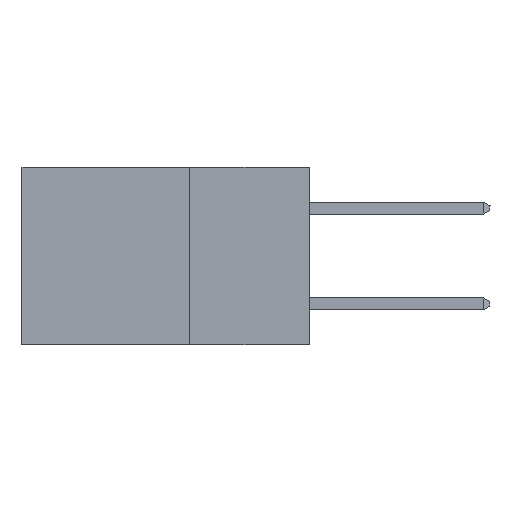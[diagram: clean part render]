
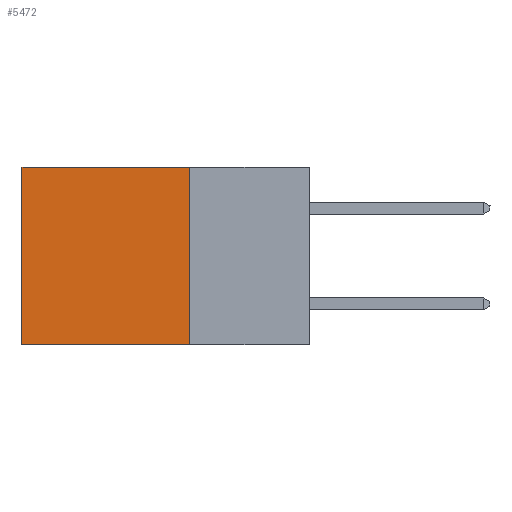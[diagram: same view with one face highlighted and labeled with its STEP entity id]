
A CAD part, left-side view. The second image highlights one B-rep face of the part: STEP entity #5472.
In plain terms, the highlighted planar face has unit normal (-1, 0, 0).
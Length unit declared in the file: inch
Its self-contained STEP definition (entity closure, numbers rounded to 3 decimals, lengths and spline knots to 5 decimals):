
#203 = LINE ( 'NONE', #6401, #4973 ) ;
#1216 = CARTESIAN_POINT ( 'NONE',  ( 0.2875, 0.25, -0.37 ) ) ;
#1405 = VERTEX_POINT ( 'NONE', #10408 ) ;
#1836 = CARTESIAN_POINT ( 'NONE',  ( 0.2875, 0.25, 0. ) ) ;
#1982 = DIRECTION ( 'NONE',  ( 1., 0., 0. ) ) ;
#2124 = VECTOR ( 'NONE', #11197, 39.37008 ) ;
#3641 = ORIENTED_EDGE ( 'NONE', *, *, #13213, .F. ) ;
#3647 = DIRECTION ( 'NONE',  ( 0., 0., -1. ) ) ;
#4337 = LINE ( 'NONE', #4484, #15552 ) ;
#4481 = VERTEX_POINT ( 'NONE', #12967 ) ;
#4484 = CARTESIAN_POINT ( 'NONE',  ( 0.2875, 0.25, 0. ) ) ;
#4973 = VECTOR ( 'NONE', #3647, 39.37008 ) ;
#5383 = EDGE_CURVE ( 'NONE', #10012, #4481, #13085, .T. ) ;
#5472 = ADVANCED_FACE ( 'NONE', ( #8079 ), #13011, .F. ) ;
#6213 = LINE ( 'NONE', #8777, #2124 ) ;
#6401 = CARTESIAN_POINT ( 'NONE',  ( 0.2875, 0.6, 0. ) ) ;
#6729 = DIRECTION ( 'NONE',  ( 0., 0., -1. ) ) ;
#7143 = EDGE_CURVE ( 'NONE', #7684, #1405, #6213, .T. ) ;
#7684 = VERTEX_POINT ( 'NONE', #1216 ) ;
#7957 = AXIS2_PLACEMENT_3D ( 'NONE', #1836, #1982, #6729 ) ;
#8079 = FACE_OUTER_BOUND ( 'NONE', #12293, .T. ) ;
#8777 = CARTESIAN_POINT ( 'NONE',  ( 0.2875, 0.25, -0.37 ) ) ;
#8874 = ORIENTED_EDGE ( 'NONE', *, *, #10955, .T. ) ;
#9365 = CARTESIAN_POINT ( 'NONE',  ( 0.2875, 0.25, 0. ) ) ;
#10012 = VERTEX_POINT ( 'NONE', #9365 ) ;
#10408 = CARTESIAN_POINT ( 'NONE',  ( 0.2875, 0.6, -0.37 ) ) ;
#10468 = ORIENTED_EDGE ( 'NONE', *, *, #7143, .F. ) ;
#10589 = DIRECTION ( 'NONE',  ( 0., 1., 0. ) ) ;
#10790 = VECTOR ( 'NONE', #10589, 39.37008 ) ;
#10955 = EDGE_CURVE ( 'NONE', #4481, #1405, #203, .T. ) ;
#11197 = DIRECTION ( 'NONE',  ( 0., 1., 0. ) ) ;
#11875 = CARTESIAN_POINT ( 'NONE',  ( 0.2875, 0.25, 0. ) ) ;
#12293 = EDGE_LOOP ( 'NONE', ( #8874, #10468, #3641, #13228 ) ) ;
#12967 = CARTESIAN_POINT ( 'NONE',  ( 0.2875, 0.6, 0. ) ) ;
#13011 = PLANE ( 'NONE',  #7957 ) ;
#13085 = LINE ( 'NONE', #11875, #10790 ) ;
#13213 = EDGE_CURVE ( 'NONE', #10012, #7684, #4337, .T. ) ;
#13228 = ORIENTED_EDGE ( 'NONE', *, *, #5383, .T. ) ;
#14218 = DIRECTION ( 'NONE',  ( 0., 0., -1. ) ) ;
#15552 = VECTOR ( 'NONE', #14218, 39.37008 ) ;
